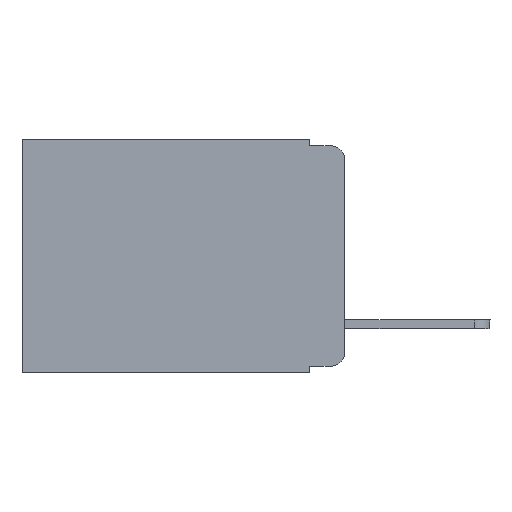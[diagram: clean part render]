
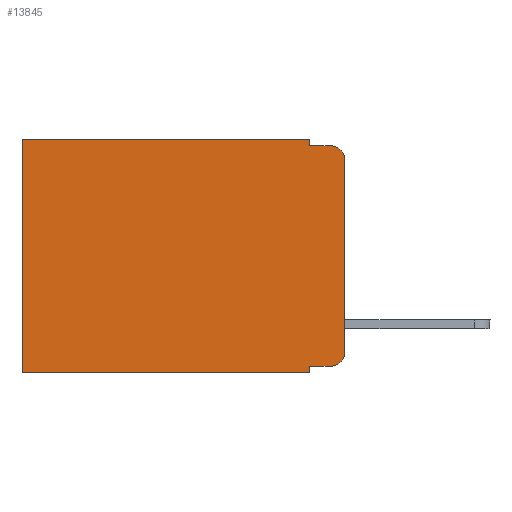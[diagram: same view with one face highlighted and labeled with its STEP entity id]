
A CAD part, left-side view. The second image highlights one B-rep face of the part: STEP entity #13845.
In plain terms, the highlighted planar face has unit normal (-1, 0, 0).
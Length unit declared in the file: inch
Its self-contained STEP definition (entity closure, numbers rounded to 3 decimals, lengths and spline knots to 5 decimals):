
#72 = VERTEX_POINT ( 'NONE', #8352 ) ;
#408 = CARTESIAN_POINT ( 'NONE',  ( 0.298, 0.051, 0. ) ) ;
#703 = CARTESIAN_POINT ( 'NONE',  ( 0.298, 0.473, 0. ) ) ;
#745 = EDGE_CURVE ( 'NONE', #2160, #21185, #23963, .T. ) ;
#1148 = VECTOR ( 'NONE', #3863, 39.37008 ) ;
#1260 = ORIENTED_EDGE ( 'NONE', *, *, #5685, .F. ) ;
#1508 = EDGE_CURVE ( 'NONE', #19670, #4591, #14595, .T. ) ;
#1651 = FACE_OUTER_BOUND ( 'NONE', #15739, .T. ) ;
#1809 = VECTOR ( 'NONE', #18484, 39.37008 ) ;
#1876 = LINE ( 'NONE', #20177, #2719 ) ;
#2001 = DIRECTION ( 'NONE',  ( 1., 0., 0. ) ) ;
#2148 = DIRECTION ( 'NONE',  ( 0., 0., -1. ) ) ;
#2160 = VERTEX_POINT ( 'NONE', #11309 ) ;
#2719 = VECTOR ( 'NONE', #18162, 39.37008 ) ;
#2741 = VECTOR ( 'NONE', #7136, 39.37008 ) ;
#3381 = ORIENTED_EDGE ( 'NONE', *, *, #23618, .T. ) ;
#3527 = ORIENTED_EDGE ( 'NONE', *, *, #12106, .F. ) ;
#3578 = CARTESIAN_POINT ( 'NONE',  ( 0.298, 0.051, -0.01 ) ) ;
#3699 = ORIENTED_EDGE ( 'NONE', *, *, #18689, .T. ) ;
#3863 = DIRECTION ( 'NONE',  ( 0., 0., -1. ) ) ;
#4023 = ORIENTED_EDGE ( 'NONE', *, *, #8287, .F. ) ;
#4452 = EDGE_CURVE ( 'NONE', #6991, #72, #23630, .T. ) ;
#4551 = CARTESIAN_POINT ( 'NONE',  ( 0.298, 0., 0. ) ) ;
#4591 = VERTEX_POINT ( 'NONE', #20386 ) ;
#4979 = AXIS2_PLACEMENT_3D ( 'NONE', #18463, #23694, #18147 ) ;
#5443 = LINE ( 'NONE', #408, #1148 ) ;
#5685 = EDGE_CURVE ( 'NONE', #20222, #21185, #18630, .T. ) ;
#5815 = ORIENTED_EDGE ( 'NONE', *, *, #4452, .F. ) ;
#6672 = LINE ( 'NONE', #9639, #1809 ) ;
#6991 = VERTEX_POINT ( 'NONE', #3578 ) ;
#7070 = DIRECTION ( 'NONE',  ( 0., -1., 0. ) ) ;
#7136 = DIRECTION ( 'NONE',  ( 0., 0., -1. ) ) ;
#7185 = CARTESIAN_POINT ( 'NONE',  ( 0.298, 0.051, -0.333 ) ) ;
#7404 = CARTESIAN_POINT ( 'NONE',  ( 0.298, 0., -0.313 ) ) ;
#7417 = VECTOR ( 'NONE', #2148, 39.37008 ) ;
#7599 = DIRECTION ( 'NONE',  ( 0., 0., -1. ) ) ;
#8287 = EDGE_CURVE ( 'NONE', #11908, #4591, #6672, .T. ) ;
#8352 = CARTESIAN_POINT ( 'NONE',  ( 0.298, 0.02, -0.01 ) ) ;
#8661 = CARTESIAN_POINT ( 'NONE',  ( 0.298, 0.051, 0. ) ) ;
#8772 = PLANE ( 'NONE',  #10604 ) ;
#9127 = CARTESIAN_POINT ( 'NONE',  ( 0.298, 0.051, 0. ) ) ;
#9639 = CARTESIAN_POINT ( 'NONE',  ( 0.298, 0., -0.343 ) ) ;
#10186 = ORIENTED_EDGE ( 'NONE', *, *, #16297, .F. ) ;
#10604 = AXIS2_PLACEMENT_3D ( 'NONE', #12993, #2001, #7599 ) ;
#10630 = VECTOR ( 'NONE', #7070, 39.37008 ) ;
#11309 = CARTESIAN_POINT ( 'NONE',  ( 0.298, 0.02, -0.333 ) ) ;
#11908 = VERTEX_POINT ( 'NONE', #21488 ) ;
#12106 = EDGE_CURVE ( 'NONE', #17603, #6991, #5443, .T. ) ;
#12551 = CARTESIAN_POINT ( 'NONE',  ( 0.298, 0.051, -0.01 ) ) ;
#12907 = LINE ( 'NONE', #9127, #7417 ) ;
#12993 = CARTESIAN_POINT ( 'NONE',  ( 0.298, 0., 0. ) ) ;
#13845 = ADVANCED_FACE ( 'NONE', ( #1651 ), #8772, .F. ) ;
#14146 = EDGE_CURVE ( 'NONE', #20222, #72, #16603, .T. ) ;
#14588 = VECTOR ( 'NONE', #23102, 39.37008 ) ;
#14595 = LINE ( 'NONE', #20785, #23340 ) ;
#15739 = EDGE_LOOP ( 'NONE', ( #1260, #22137, #5815, #3527, #3381, #22044, #4023, #10186, #3699, #20676 ) ) ;
#16297 = EDGE_CURVE ( 'NONE', #17220, #11908, #12907, .T. ) ;
#16603 = CIRCLE ( 'NONE', #4979, 0.02 ) ;
#16786 = AXIS2_PLACEMENT_3D ( 'NONE', #23036, #23361, #21487 ) ;
#17220 = VERTEX_POINT ( 'NONE', #7185 ) ;
#17551 = CARTESIAN_POINT ( 'NONE',  ( 0.298, 0., -0.03 ) ) ;
#17603 = VERTEX_POINT ( 'NONE', #8661 ) ;
#18127 = CARTESIAN_POINT ( 'NONE',  ( 0.298, 0., 0. ) ) ;
#18147 = DIRECTION ( 'NONE',  ( 0., 0., -1. ) ) ;
#18162 = DIRECTION ( 'NONE',  ( 0., -1., 0. ) ) ;
#18463 = CARTESIAN_POINT ( 'NONE',  ( 0.298, 0.02, -0.03 ) ) ;
#18484 = DIRECTION ( 'NONE',  ( 0., 1., 0. ) ) ;
#18630 = LINE ( 'NONE', #18127, #2741 ) ;
#18689 = EDGE_CURVE ( 'NONE', #17220, #2160, #1876, .T. ) ;
#19082 = DIRECTION ( 'NONE',  ( 0., 0., -1. ) ) ;
#19261 = LINE ( 'NONE', #4551, #14588 ) ;
#19670 = VERTEX_POINT ( 'NONE', #703 ) ;
#20177 = CARTESIAN_POINT ( 'NONE',  ( 0.298, 0.051, -0.333 ) ) ;
#20222 = VERTEX_POINT ( 'NONE', #17551 ) ;
#20386 = CARTESIAN_POINT ( 'NONE',  ( 0.298, 0.473, -0.343 ) ) ;
#20676 = ORIENTED_EDGE ( 'NONE', *, *, #745, .T. ) ;
#20785 = CARTESIAN_POINT ( 'NONE',  ( 0.298, 0.473, 0. ) ) ;
#21185 = VERTEX_POINT ( 'NONE', #7404 ) ;
#21487 = DIRECTION ( 'NONE',  ( 0., 0., -1. ) ) ;
#21488 = CARTESIAN_POINT ( 'NONE',  ( 0.298, 0.051, -0.343 ) ) ;
#22044 = ORIENTED_EDGE ( 'NONE', *, *, #1508, .T. ) ;
#22137 = ORIENTED_EDGE ( 'NONE', *, *, #14146, .T. ) ;
#23036 = CARTESIAN_POINT ( 'NONE',  ( 0.298, 0.02, -0.313 ) ) ;
#23102 = DIRECTION ( 'NONE',  ( 0., 1., 0. ) ) ;
#23340 = VECTOR ( 'NONE', #19082, 39.37008 ) ;
#23361 = DIRECTION ( 'NONE',  ( -1., 0., 0. ) ) ;
#23618 = EDGE_CURVE ( 'NONE', #17603, #19670, #19261, .T. ) ;
#23630 = LINE ( 'NONE', #12551, #10630 ) ;
#23694 = DIRECTION ( 'NONE',  ( -1., 0., 0. ) ) ;
#23963 = CIRCLE ( 'NONE', #16786, 0.02 ) ;
